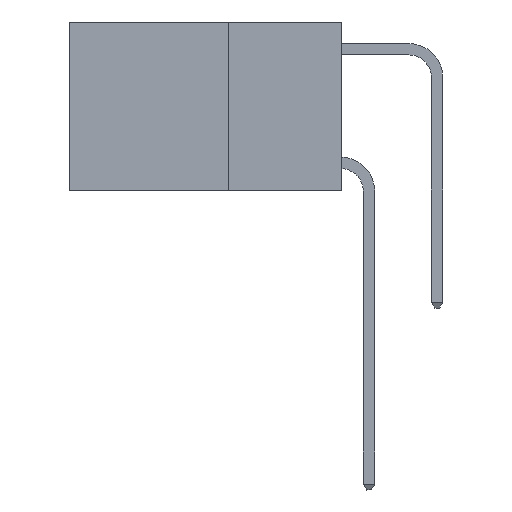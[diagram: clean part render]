
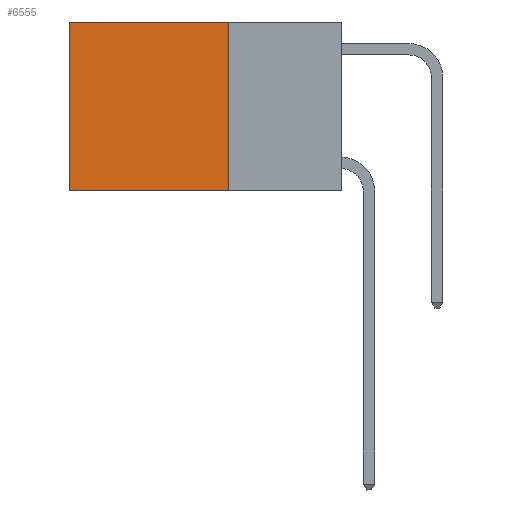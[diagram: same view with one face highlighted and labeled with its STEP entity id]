
A CAD part, left-side view. The second image highlights one B-rep face of the part: STEP entity #6555.
In plain terms, the highlighted planar face has unit normal (-1, 0, 0).
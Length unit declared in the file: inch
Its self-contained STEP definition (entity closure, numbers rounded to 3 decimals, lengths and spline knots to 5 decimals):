
#392 = CARTESIAN_POINT ( 'NONE',  ( 0.2625, 0.25, 0. ) ) ;
#1423 = VECTOR ( 'NONE', #2894, 39.37008 ) ;
#1838 = ORIENTED_EDGE ( 'NONE', *, *, #9945, .T. ) ;
#2147 = ORIENTED_EDGE ( 'NONE', *, *, #10807, .F. ) ;
#2248 = CARTESIAN_POINT ( 'NONE',  ( 0.2625, 0.25, 0. ) ) ;
#2288 = ORIENTED_EDGE ( 'NONE', *, *, #12801, .T. ) ;
#2894 = DIRECTION ( 'NONE',  ( 0., 1., 0. ) ) ;
#3069 = VERTEX_POINT ( 'NONE', #11659 ) ;
#3632 = PLANE ( 'NONE',  #4757 ) ;
#4737 = VERTEX_POINT ( 'NONE', #10202 ) ;
#4757 = AXIS2_PLACEMENT_3D ( 'NONE', #392, #10849, #12222 ) ;
#5375 = DIRECTION ( 'NONE',  ( 0., 1., 0. ) ) ;
#5377 = VECTOR ( 'NONE', #13999, 39.37008 ) ;
#5830 = VERTEX_POINT ( 'NONE', #10990 ) ;
#6034 = VECTOR ( 'NONE', #9863, 39.37008 ) ;
#6476 = CARTESIAN_POINT ( 'NONE',  ( 0.2625, 0.6, 0. ) ) ;
#6555 = ADVANCED_FACE ( 'NONE', ( #13770 ), #3632, .F. ) ;
#7397 = CARTESIAN_POINT ( 'NONE',  ( 0.2625, 0.6, 0. ) ) ;
#8164 = CARTESIAN_POINT ( 'NONE',  ( 0.2625, 0.25, 0. ) ) ;
#9475 = LINE ( 'NONE', #2248, #17914 ) ;
#9863 = DIRECTION ( 'NONE',  ( 0., 0., -1. ) ) ;
#9945 = EDGE_CURVE ( 'NONE', #5830, #12208, #9475, .T. ) ;
#10202 = CARTESIAN_POINT ( 'NONE',  ( 0.2625, 0.25, -0.37 ) ) ;
#10807 = EDGE_CURVE ( 'NONE', #5830, #4737, #12644, .T. ) ;
#10849 = DIRECTION ( 'NONE',  ( 1., 0., 0. ) ) ;
#10990 = CARTESIAN_POINT ( 'NONE',  ( 0.2625, 0.25, 0. ) ) ;
#11659 = CARTESIAN_POINT ( 'NONE',  ( 0.2625, 0.6, -0.37 ) ) ;
#12208 = VERTEX_POINT ( 'NONE', #6476 ) ;
#12222 = DIRECTION ( 'NONE',  ( 0., 0., -1. ) ) ;
#12258 = ORIENTED_EDGE ( 'NONE', *, *, #18457, .F. ) ;
#12644 = LINE ( 'NONE', #8164, #5377 ) ;
#12704 = EDGE_LOOP ( 'NONE', ( #2288, #12258, #2147, #1838 ) ) ;
#12801 = EDGE_CURVE ( 'NONE', #12208, #3069, #15794, .T. ) ;
#13137 = LINE ( 'NONE', #18988, #1423 ) ;
#13770 = FACE_OUTER_BOUND ( 'NONE', #12704, .T. ) ;
#13999 = DIRECTION ( 'NONE',  ( 0., 0., -1. ) ) ;
#15794 = LINE ( 'NONE', #7397, #6034 ) ;
#17914 = VECTOR ( 'NONE', #5375, 39.37008 ) ;
#18457 = EDGE_CURVE ( 'NONE', #4737, #3069, #13137, .T. ) ;
#18988 = CARTESIAN_POINT ( 'NONE',  ( 0.2625, 0.25, -0.37 ) ) ;
